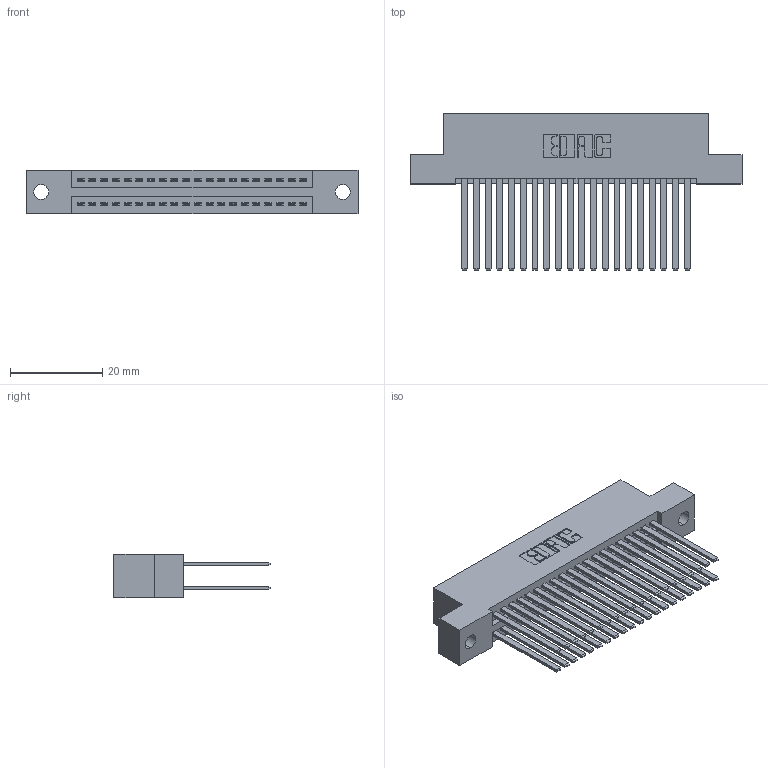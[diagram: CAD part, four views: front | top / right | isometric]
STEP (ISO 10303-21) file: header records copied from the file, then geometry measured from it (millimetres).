
FILE_DESCRIPTION (( 'STEP AP203' ), '1' );
FILE_NAME ('395-040-544-202.STEP', '2019-10-18T05:39:23', ( '' ), ( '' ), 'SwSTEP 2.0', 'SolidWorks 2016', '' );
FILE_SCHEMA (( 'CONFIG_CONTROL_DESIGN' ));
Length unit declared in the file: inch
Products named in the file (3): 345 Part_Flush Mounting Lugs - 0.128 Dia; 345-292-001_345-293-144; 395-040-544-202
Assembly tree (41 placements, depth 2):
  395-040-544-202
    345 Part_Flush Mounting Lugs - 0.128 Dia
    345-292-001_345-293-144  x40
Bounding box: 72.01 x 33.96 x 9.4 mm (x, y, z)
Volume: 7314.9 mm3; surface area: 11757.2 mm2
Topology: 41 solids, 41 shells, 1886 faces, 5581 edges, 3666 vertices
Faces by surface type: plane 1240, cylinder 646
Entity records: 18473 total; most frequent: CARTESIAN_POINT 3116, ORIENTED_EDGE 3050, DIRECTION 2773, EDGE_CURVE 1525, LINE 1317, VECTOR 1317, VERTEX_POINT 1014, AXIS2_PLACEMENT_3D 728
